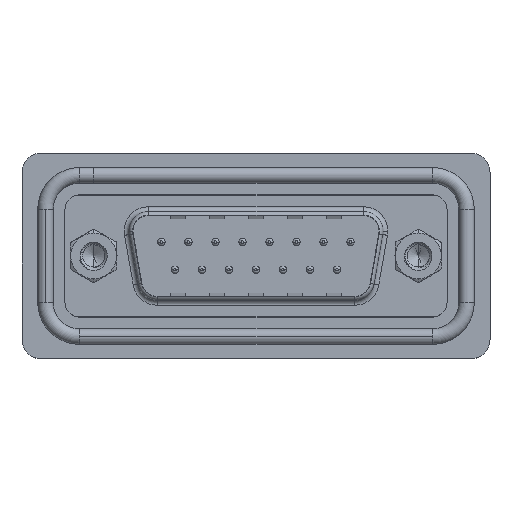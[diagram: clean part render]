
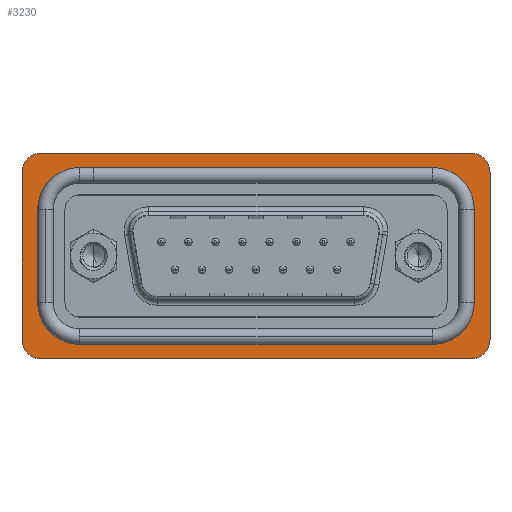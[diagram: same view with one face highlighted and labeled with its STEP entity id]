
A CAD part, top view. The second image highlights one B-rep face of the part: STEP entity #3230.
In plain terms, the highlighted planar face has unit normal (0, 0, 1).
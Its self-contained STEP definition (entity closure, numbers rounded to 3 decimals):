
#74 = CARTESIAN_POINT ( 'NONE',  ( 40.65, -8.55, 0.5 ) ) ;
#375 = CARTESIAN_POINT ( 'NONE',  ( 38.65, 10.55, 0.5 ) ) ;
#418 = EDGE_CURVE ( 'NONE', #22070, #11241, #11030, .T. ) ;
#421 = CIRCLE ( 'NONE', #2332, 4.3 ) ;
#1172 = DIRECTION ( 'NONE',  ( 1., 0., 0. ) ) ;
#1432 = CARTESIAN_POINT ( 'NONE',  ( -7.35, 8.55, 0.5 ) ) ;
#1898 = LINE ( 'NONE', #14744, #11662 ) ;
#1951 = DIRECTION ( 'NONE',  ( 0., 0., 1. ) ) ;
#2308 = EDGE_CURVE ( 'NONE', #19191, #22070, #2467, .T. ) ;
#2332 = AXIS2_PLACEMENT_3D ( 'NONE', #20227, #1951, #9045 ) ;
#2339 = ORIENTED_EDGE ( 'NONE', *, *, #21191, .T. ) ;
#2467 = LINE ( 'NONE', #9680, #23187 ) ;
#2843 = PLANE ( 'NONE',  #3225 ) ;
#3225 = AXIS2_PLACEMENT_3D ( 'NONE', #6510, #8392, #21013 ) ;
#3230 = ADVANCED_FACE ( 'NONE', ( #13701, #13363 ), #2843, .T. ) ;
#3281 = CIRCLE ( 'NONE', #14583, 2. ) ;
#3497 = ORIENTED_EDGE ( 'NONE', *, *, #17192, .T. ) ;
#3644 = DIRECTION ( 'NONE',  ( 1., 0., 0. ) ) ;
#3648 = CARTESIAN_POINT ( 'NONE',  ( 40.65, 8.55, 0.5 ) ) ;
#4278 = CARTESIAN_POINT ( 'NONE',  ( 34.745, -9.075, 0.5 ) ) ;
#4351 = DIRECTION ( 'NONE',  ( 0., 1., 0. ) ) ;
#4440 = DIRECTION ( 'NONE',  ( 1., 0., 0. ) ) ;
#4543 = CIRCLE ( 'NONE', #17714, 2. ) ;
#4649 = DIRECTION ( 'NONE',  ( 0., 0., 1. ) ) ;
#4661 = VERTEX_POINT ( 'NONE', #7050 ) ;
#4742 = ORIENTED_EDGE ( 'NONE', *, *, #20797, .T. ) ;
#5098 = CIRCLE ( 'NONE', #15267, 2. ) ;
#5153 = CARTESIAN_POINT ( 'NONE',  ( -5.35, 10.55, 0.5 ) ) ;
#5517 = CIRCLE ( 'NONE', #16081, 4.3 ) ;
#5618 = VECTOR ( 'NONE', #6483, 1000. ) ;
#5828 = CARTESIAN_POINT ( 'NONE',  ( -7.35, -8.55, 0.5 ) ) ;
#6072 = VECTOR ( 'NONE', #7518, 1000. ) ;
#6129 = ORIENTED_EDGE ( 'NONE', *, *, #23003, .T. ) ;
#6382 = VERTEX_POINT ( 'NONE', #375 ) ;
#6450 = VERTEX_POINT ( 'NONE', #4278 ) ;
#6483 = DIRECTION ( 'NONE',  ( -1., 0., 0. ) ) ;
#6510 = CARTESIAN_POINT ( 'NONE',  ( 38.65, 8.55, 0.5 ) ) ;
#6594 = CARTESIAN_POINT ( 'NONE',  ( 34.745, 9.075, 0.5 ) ) ;
#6616 = VERTEX_POINT ( 'NONE', #22681 ) ;
#6753 = VERTEX_POINT ( 'NONE', #1432 ) ;
#6809 = VERTEX_POINT ( 'NONE', #3648 ) ;
#6872 = EDGE_CURVE ( 'NONE', #6616, #6450, #1898, .T. ) ;
#6968 = EDGE_CURVE ( 'NONE', #11241, #16485, #13578, .T. ) ;
#7050 = CARTESIAN_POINT ( 'NONE',  ( -5.745, 4.775, 0.5 ) ) ;
#7077 = DIRECTION ( 'NONE',  ( 0., 0., 1. ) ) ;
#7394 = LINE ( 'NONE', #74, #6072 ) ;
#7518 = DIRECTION ( 'NONE',  ( 0., 1., 0. ) ) ;
#7553 = DIRECTION ( 'NONE',  ( 1., 0., 0. ) ) ;
#7873 = DIRECTION ( 'NONE',  ( 0., 0., 1. ) ) ;
#7927 = CARTESIAN_POINT ( 'NONE',  ( 40.65, -8.55, 0.5 ) ) ;
#7990 = ORIENTED_EDGE ( 'NONE', *, *, #6872, .F. ) ;
#8167 = VERTEX_POINT ( 'NONE', #22536 ) ;
#8306 = ORIENTED_EDGE ( 'NONE', *, *, #17614, .T. ) ;
#8392 = DIRECTION ( 'NONE',  ( 0., 0., 1. ) ) ;
#8512 = VECTOR ( 'NONE', #16915, 1000. ) ;
#8689 = CARTESIAN_POINT ( 'NONE',  ( 38.65, 10.55, 0.5 ) ) ;
#8726 = CARTESIAN_POINT ( 'NONE',  ( -5.745, 4.775, 0.5 ) ) ;
#8760 = VERTEX_POINT ( 'NONE', #19645 ) ;
#8876 = LINE ( 'NONE', #9220, #10052 ) ;
#9045 = DIRECTION ( 'NONE',  ( 1., 0., 0. ) ) ;
#9136 = LINE ( 'NONE', #5828, #8512 ) ;
#9220 = CARTESIAN_POINT ( 'NONE',  ( 38.65, -10.55, 0.5 ) ) ;
#9556 = CARTESIAN_POINT ( 'NONE',  ( -5.745, -4.775, 0.5 ) ) ;
#9576 = EDGE_CURVE ( 'NONE', #6809, #6382, #4543, .T. ) ;
#9605 = CARTESIAN_POINT ( 'NONE',  ( 34.745, 9.075, 0.5 ) ) ;
#9680 = CARTESIAN_POINT ( 'NONE',  ( 39.045, -4.775, 0.5 ) ) ;
#9798 = CARTESIAN_POINT ( 'NONE',  ( -1.445, 9.075, 0.5 ) ) ;
#10025 = CARTESIAN_POINT ( 'NONE',  ( -5.35, -10.55, 0.5 ) ) ;
#10052 = VECTOR ( 'NONE', #14635, 1000. ) ;
#10101 = EDGE_CURVE ( 'NONE', #14752, #6809, #7394, .T. ) ;
#10309 = DIRECTION ( 'NONE',  ( 1., 0., 0. ) ) ;
#10428 = CARTESIAN_POINT ( 'NONE',  ( 38.65, 8.55, 0.5 ) ) ;
#10615 = DIRECTION ( 'NONE',  ( 0., 0., 1. ) ) ;
#10679 = EDGE_CURVE ( 'NONE', #13679, #6616, #421, .T. ) ;
#10834 = AXIS2_PLACEMENT_3D ( 'NONE', #20999, #10615, #1172 ) ;
#11030 = CIRCLE ( 'NONE', #18553, 4.3 ) ;
#11241 = VERTEX_POINT ( 'NONE', #9605 ) ;
#11532 = DIRECTION ( 'NONE',  ( 1., 0., 0. ) ) ;
#11584 = ORIENTED_EDGE ( 'NONE', *, *, #20035, .T. ) ;
#11662 = VECTOR ( 'NONE', #7553, 1000. ) ;
#11989 = LINE ( 'NONE', #8689, #21734 ) ;
#12302 = AXIS2_PLACEMENT_3D ( 'NONE', #22374, #7873, #11532 ) ;
#12372 = LINE ( 'NONE', #8726, #17894 ) ;
#12592 = ORIENTED_EDGE ( 'NONE', *, *, #418, .F. ) ;
#12973 = EDGE_LOOP ( 'NONE', ( #14177, #3497, #6129, #4742, #11584, #2339, #8306, #14792 ) ) ;
#13363 = FACE_OUTER_BOUND ( 'NONE', #12973, .T. ) ;
#13418 = CARTESIAN_POINT ( 'NONE',  ( 34.745, 4.775, 0.5 ) ) ;
#13515 = CARTESIAN_POINT ( 'NONE',  ( 39.045, 4.775, 0.5 ) ) ;
#13578 = LINE ( 'NONE', #6594, #5618 ) ;
#13679 = VERTEX_POINT ( 'NONE', #9556 ) ;
#13701 = FACE_BOUND ( 'NONE', #22683, .T. ) ;
#13943 = VERTEX_POINT ( 'NONE', #5153 ) ;
#13985 = DIRECTION ( 'NONE',  ( -1., 0., 0. ) ) ;
#14038 = ORIENTED_EDGE ( 'NONE', *, *, #17079, .F. ) ;
#14177 = ORIENTED_EDGE ( 'NONE', *, *, #9576, .T. ) ;
#14583 = AXIS2_PLACEMENT_3D ( 'NONE', #21361, #7077, #3644 ) ;
#14635 = DIRECTION ( 'NONE',  ( 1., 0., 0. ) ) ;
#14744 = CARTESIAN_POINT ( 'NONE',  ( -1.445, -9.075, 0.5 ) ) ;
#14752 = VERTEX_POINT ( 'NONE', #7927 ) ;
#14792 = ORIENTED_EDGE ( 'NONE', *, *, #10101, .T. ) ;
#15267 = AXIS2_PLACEMENT_3D ( 'NONE', #20529, #20169, #18522 ) ;
#15401 = ORIENTED_EDGE ( 'NONE', *, *, #17358, .F. ) ;
#15730 = CIRCLE ( 'NONE', #10834, 2. ) ;
#16081 = AXIS2_PLACEMENT_3D ( 'NONE', #20100, #18459, #17975 ) ;
#16343 = DIRECTION ( 'NONE',  ( 0., -1., 0. ) ) ;
#16485 = VERTEX_POINT ( 'NONE', #9798 ) ;
#16502 = VERTEX_POINT ( 'NONE', #10025 ) ;
#16915 = DIRECTION ( 'NONE',  ( 0., -1., 0. ) ) ;
#17079 = EDGE_CURVE ( 'NONE', #16485, #4661, #22477, .T. ) ;
#17192 = EDGE_CURVE ( 'NONE', #6382, #13943, #11989, .T. ) ;
#17358 = EDGE_CURVE ( 'NONE', #6450, #19191, #5517, .T. ) ;
#17614 = EDGE_CURVE ( 'NONE', #8167, #14752, #3281, .T. ) ;
#17714 = AXIS2_PLACEMENT_3D ( 'NONE', #10428, #4649, #10309 ) ;
#17894 = VECTOR ( 'NONE', #16343, 1000. ) ;
#17975 = DIRECTION ( 'NONE',  ( 1., 0., 0. ) ) ;
#18459 = DIRECTION ( 'NONE',  ( 0., 0., 1. ) ) ;
#18486 = ORIENTED_EDGE ( 'NONE', *, *, #6968, .F. ) ;
#18522 = DIRECTION ( 'NONE',  ( -1., 0., 0. ) ) ;
#18553 = AXIS2_PLACEMENT_3D ( 'NONE', #13418, #20601, #4440 ) ;
#18904 = ORIENTED_EDGE ( 'NONE', *, *, #20316, .F. ) ;
#19191 = VERTEX_POINT ( 'NONE', #21051 ) ;
#19645 = CARTESIAN_POINT ( 'NONE',  ( -7.35, -8.55, 0.5 ) ) ;
#20035 = EDGE_CURVE ( 'NONE', #8760, #16502, #5098, .T. ) ;
#20100 = CARTESIAN_POINT ( 'NONE',  ( 34.745, -4.775, 0.5 ) ) ;
#20169 = DIRECTION ( 'NONE',  ( 0., 0., 1. ) ) ;
#20227 = CARTESIAN_POINT ( 'NONE',  ( -1.445, -4.775, 0.5 ) ) ;
#20316 = EDGE_CURVE ( 'NONE', #4661, #13679, #12372, .T. ) ;
#20529 = CARTESIAN_POINT ( 'NONE',  ( -5.35, -8.55, 0.5 ) ) ;
#20601 = DIRECTION ( 'NONE',  ( 0., 0., 1. ) ) ;
#20797 = EDGE_CURVE ( 'NONE', #6753, #8760, #9136, .T. ) ;
#20864 = ORIENTED_EDGE ( 'NONE', *, *, #10679, .F. ) ;
#20999 = CARTESIAN_POINT ( 'NONE',  ( -5.35, 8.55, 0.5 ) ) ;
#21013 = DIRECTION ( 'NONE',  ( 1., 0., 0. ) ) ;
#21051 = CARTESIAN_POINT ( 'NONE',  ( 39.045, -4.775, 0.5 ) ) ;
#21191 = EDGE_CURVE ( 'NONE', #16502, #8167, #8876, .T. ) ;
#21361 = CARTESIAN_POINT ( 'NONE',  ( 38.65, -8.55, 0.5 ) ) ;
#21734 = VECTOR ( 'NONE', #13985, 1000. ) ;
#22070 = VERTEX_POINT ( 'NONE', #13515 ) ;
#22354 = ORIENTED_EDGE ( 'NONE', *, *, #2308, .F. ) ;
#22374 = CARTESIAN_POINT ( 'NONE',  ( -1.445, 4.775, 0.5 ) ) ;
#22477 = CIRCLE ( 'NONE', #12302, 4.3 ) ;
#22536 = CARTESIAN_POINT ( 'NONE',  ( 38.65, -10.55, 0.5 ) ) ;
#22681 = CARTESIAN_POINT ( 'NONE',  ( -1.445, -9.075, 0.5 ) ) ;
#22683 = EDGE_LOOP ( 'NONE', ( #12592, #22354, #15401, #7990, #20864, #18904, #14038, #18486 ) ) ;
#23003 = EDGE_CURVE ( 'NONE', #13943, #6753, #15730, .T. ) ;
#23187 = VECTOR ( 'NONE', #4351, 1000. ) ;
